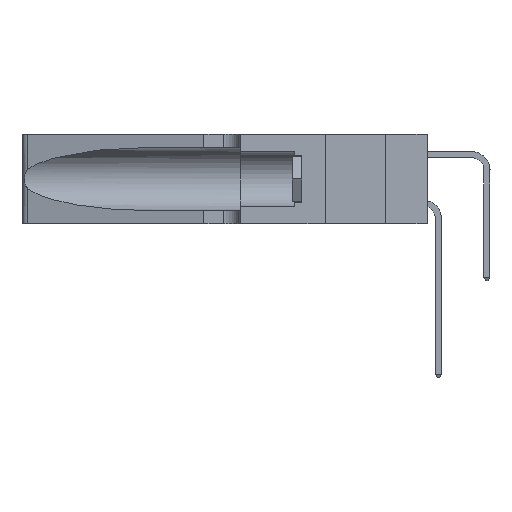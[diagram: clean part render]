
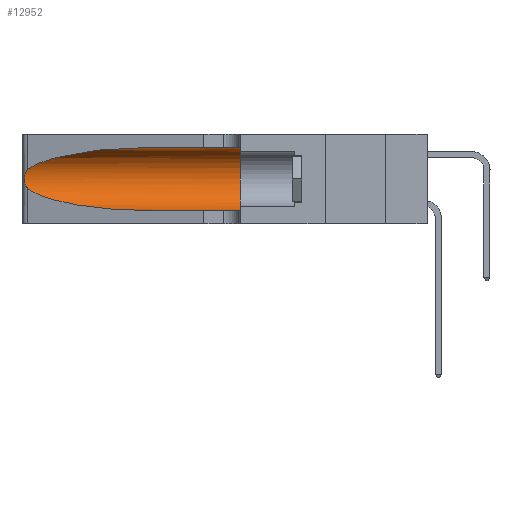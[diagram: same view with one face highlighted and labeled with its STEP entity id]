
A CAD part, left-side view. The second image highlights one B-rep face of the part: STEP entity #12952.
In plain terms, the highlighted cylindrical face has radius 3.308 mm (diameter 6.617 mm), a partial arc.
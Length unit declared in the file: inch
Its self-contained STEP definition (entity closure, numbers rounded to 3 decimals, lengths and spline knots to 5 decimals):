
#207 = LINE ( 'NONE', #33569, #38886 ) ;
#244 = CARTESIAN_POINT ( 'NONE',  ( 0.25487, 1.22718, 0.22369 ) ) ;
#1871 = DIRECTION ( 'NONE',  ( 0., 1., 0. ) ) ;
#2846 = FACE_OUTER_BOUND ( 'NONE', #38126, .T. ) ;
#3402 = CARTESIAN_POINT ( 'NONE',  ( 0.25854, 1.2359, 0.20912 ) ) ;
#3861 = EDGE_CURVE ( 'NONE', #39112, #19544, #22922, .T. ) ;
#6300 = CARTESIAN_POINT ( 'NONE',  ( 0.2373, 1.15595, 0.08982 ) ) ;
#6490 = CARTESIAN_POINT ( 'NONE',  ( 0.26075, 1.23896, 0.19203 ) ) ;
#6502 = VERTEX_POINT ( 'NONE', #26778 ) ;
#7291 = EDGE_CURVE ( 'NONE', #33029, #37171, #207, .T. ) ;
#8275 = ORIENTED_EDGE ( 'NONE', *, *, #16625, .F. ) ;
#9039 = CARTESIAN_POINT ( 'NONE',  ( 0.1305, 1.61858, 0.185 ) ) ;
#9355 = VECTOR ( 'NONE', #14634, 39.37008 ) ;
#9635 = CARTESIAN_POINT ( 'NONE',  ( 0.26017, 1.23833, 0.17102 ) ) ;
#9963 = EDGE_CURVE ( 'NONE', #10462, #39112, #21959, .T. ) ;
#10462 = VERTEX_POINT ( 'NONE', #14732 ) ;
#11053 = ORIENTED_EDGE ( 'NONE', *, *, #20848, .T. ) ;
#11227 = ORIENTED_EDGE ( 'NONE', *, *, #3861, .T. ) ;
#11368 = CARTESIAN_POINT ( 'NONE',  ( 0.1305, 0.72297, 0.05475 ) ) ;
#11529 = CARTESIAN_POINT ( 'NONE',  ( 0.1305, 1.61858, 0.31525 ) ) ;
#12426 = ORIENTED_EDGE ( 'NONE', *, *, #9963, .T. ) ;
#12523 = CARTESIAN_POINT ( 'NONE',  ( 0.1305, 0.72297, 0.05475 ) ) ;
#12723 = CARTESIAN_POINT ( 'NONE',  ( 0.25789, 1.23486, 0.15765 ) ) ;
#12952 = ADVANCED_FACE ( 'NONE', ( #2846 ), #18781, .F. ) ;
#14634 = DIRECTION ( 'NONE',  ( 0., -1., 0. ) ) ;
#14732 = CARTESIAN_POINT ( 'NONE',  ( 0.1305, 0.72297, 0.31525 ) ) ;
#15470 = CARTESIAN_POINT ( 'NONE',  ( 0.25487, 1.22718, 0.14631 ) ) ;
#15653 = CARTESIAN_POINT ( 'NONE',  ( 0.25639, 1.23184, 0.21858 ) ) ;
#15789 = CARTESIAN_POINT ( 'NONE',  ( 0.25555, 1.22993, 0.14849 ) ) ;
#16625 = EDGE_CURVE ( 'NONE', #6502, #37171, #35609, .T. ) ;
#18370 = CARTESIAN_POINT ( 'NONE',  ( 0.2373, 1.15595, 0.28018 ) ) ;
#18712 = CARTESIAN_POINT ( 'NONE',  ( 0.25555, 1.22994, 0.2215 ) ) ;
#18781 = CYLINDRICAL_SURFACE ( 'NONE', #31747, 0.13025 ) ;
#19544 = VERTEX_POINT ( 'NONE', #33079 ) ;
#19730 =( BOUNDED_CURVE ( )  B_SPLINE_CURVE ( 3, ( #15470, #6300, #30768, #12523 ),
 .UNSPECIFIED., .F., .T. ) 
 B_SPLINE_CURVE_WITH_KNOTS ( ( 4, 4 ),
 ( 3.44316, 4.71239 ),
 .UNSPECIFIED. ) 
 CURVE ( )  GEOMETRIC_REPRESENTATION_ITEM ( )  RATIONAL_B_SPLINE_CURVE ( ( 1., 0.87, 0.87, 1. ) ) 
 REPRESENTATION_ITEM ( '' )  );
#20309 = CARTESIAN_POINT ( 'NONE',  ( 0.1305, 0.35, 0.185 ) ) ;
#20510 = CARTESIAN_POINT ( 'NONE',  ( 0.25487, 1.22718, 0.22369 ) ) ;
#20627 = AXIS2_PLACEMENT_3D ( 'NONE', #20309, #1871, #23414 ) ;
#20848 = EDGE_CURVE ( 'NONE', #19544, #33029, #19730, .T. ) ;
#21802 = CARTESIAN_POINT ( 'NONE',  ( 0.25787, 1.23484, 0.2124 ) ) ;
#21959 =( BOUNDED_CURVE ( )  B_SPLINE_CURVE ( 3, ( #33238, #39400, #18370, #39521 ),
 .UNSPECIFIED., .F., .F. ) 
 B_SPLINE_CURVE_WITH_KNOTS ( ( 4, 4 ),
 ( 1.5708, 2.84003 ),
 .UNSPECIFIED. ) 
 CURVE ( )  GEOMETRIC_REPRESENTATION_ITEM ( )  RATIONAL_B_SPLINE_CURVE ( ( 1., 0.87, 0.87, 1. ) ) 
 REPRESENTATION_ITEM ( '' )  );
#22922 = B_SPLINE_CURVE_WITH_KNOTS ( 'NONE', 3,
 ( #244, #18712, #15653, #21802, #3402, #24865, #6490, #27934, #9635, #30948, #12723, #33982, #15789, #37000 ),
 .UNSPECIFIED., .F., .F.,
 ( 4, 2, 2, 2, 2, 2, 4 ),
 ( 0., 0.00027, 0.00053, 0.00107, 0.0016, 0.00187, 0.00214 ),
 .UNSPECIFIED. ) ;
#23414 = DIRECTION ( 'NONE',  ( 0., 0., 1. ) ) ;
#24285 = DIRECTION ( 'NONE',  ( 0., 0., -1. ) ) ;
#24865 = CARTESIAN_POINT ( 'NONE',  ( 0.26018, 1.23835, 0.19895 ) ) ;
#26778 = CARTESIAN_POINT ( 'NONE',  ( 0.1305, 0.35, 0.31525 ) ) ;
#27934 = CARTESIAN_POINT ( 'NONE',  ( 0.26075, 1.23896, 0.178 ) ) ;
#30768 = CARTESIAN_POINT ( 'NONE',  ( 0.18966, 0.96281, 0.05475 ) ) ;
#30948 = CARTESIAN_POINT ( 'NONE',  ( 0.25856, 1.23593, 0.16098 ) ) ;
#31747 = AXIS2_PLACEMENT_3D ( 'NONE', #9039, #33269, #24285 ) ;
#31887 = EDGE_CURVE ( 'NONE', #10462, #6502, #33645, .T. ) ;
#33029 = VERTEX_POINT ( 'NONE', #11368 ) ;
#33079 = CARTESIAN_POINT ( 'NONE',  ( 0.25487, 1.22718, 0.14631 ) ) ;
#33238 = CARTESIAN_POINT ( 'NONE',  ( 0.1305, 0.72297, 0.31525 ) ) ;
#33269 = DIRECTION ( 'NONE',  ( 0., -1., 0. ) ) ;
#33569 = CARTESIAN_POINT ( 'NONE',  ( 0.1305, 1.61858, 0.05475 ) ) ;
#33645 = LINE ( 'NONE', #11529, #9355 ) ;
#33682 = ORIENTED_EDGE ( 'NONE', *, *, #31887, .F. ) ;
#33982 = CARTESIAN_POINT ( 'NONE',  ( 0.25639, 1.23186, 0.15144 ) ) ;
#35609 = CIRCLE ( 'NONE', #20627, 0.13025 ) ;
#36176 = CARTESIAN_POINT ( 'NONE',  ( 0.1305, 0.35, 0.05475 ) ) ;
#36594 = DIRECTION ( 'NONE',  ( 0., -1., 0. ) ) ;
#36756 = ORIENTED_EDGE ( 'NONE', *, *, #7291, .T. ) ;
#37000 = CARTESIAN_POINT ( 'NONE',  ( 0.25487, 1.22718, 0.14631 ) ) ;
#37171 = VERTEX_POINT ( 'NONE', #36176 ) ;
#38126 = EDGE_LOOP ( 'NONE', ( #12426, #11227, #11053, #36756, #8275, #33682 ) ) ;
#38886 = VECTOR ( 'NONE', #36594, 39.37008 ) ;
#39112 = VERTEX_POINT ( 'NONE', #20510 ) ;
#39400 = CARTESIAN_POINT ( 'NONE',  ( 0.18966, 0.96281, 0.31525 ) ) ;
#39521 = CARTESIAN_POINT ( 'NONE',  ( 0.25487, 1.22718, 0.22369 ) ) ;
